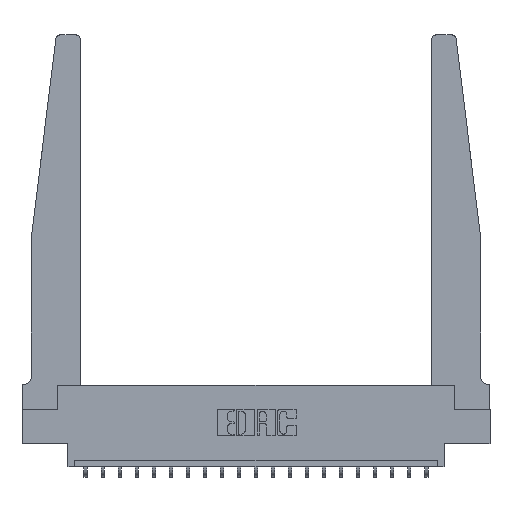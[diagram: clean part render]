
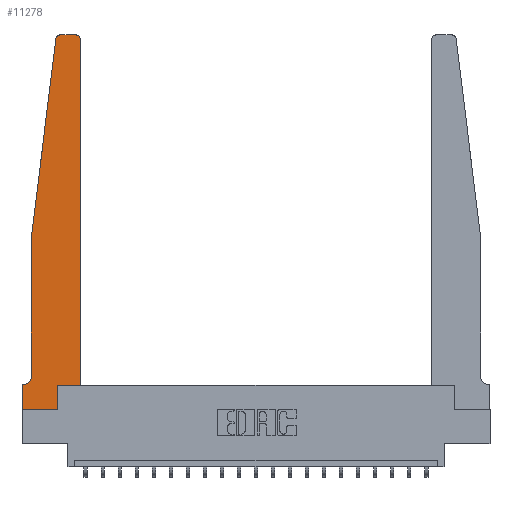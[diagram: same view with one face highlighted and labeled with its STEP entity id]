
A CAD part, top view. The second image highlights one B-rep face of the part: STEP entity #11278.
In plain terms, the highlighted planar face has unit normal (0, 0, 1).
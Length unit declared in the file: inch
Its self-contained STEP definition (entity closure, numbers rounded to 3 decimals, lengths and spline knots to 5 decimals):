
#734 = DIRECTION ( 'NONE',  ( 0., 1., 0. ) ) ;
#1067 = EDGE_CURVE ( 'NONE', #11489, #17803, #10407, .T. ) ;
#1849 = ORIENTED_EDGE ( 'NONE', *, *, #5977, .T. ) ;
#2045 = CARTESIAN_POINT ( 'NONE',  ( 0., 0., 0.37 ) ) ;
#2107 = DIRECTION ( 'NONE',  ( 0., 0., 1. ) ) ;
#2179 = ORIENTED_EDGE ( 'NONE', *, *, #11530, .T. ) ;
#2269 = AXIS2_PLACEMENT_3D ( 'NONE', #3315, #14620, #4945 ) ;
#2359 = LINE ( 'NONE', #6190, #10485 ) ;
#2527 = CARTESIAN_POINT ( 'NONE',  ( 0.2605, 0.18, 0.37 ) ) ;
#3315 = CARTESIAN_POINT ( 'NONE',  ( 0.015, 0.2375, 0.37 ) ) ;
#3487 = LINE ( 'NONE', #10428, #12092 ) ;
#3528 = CARTESIAN_POINT ( 'NONE',  ( 0.395, 2.75, 0.37 ) ) ;
#3557 = PLANE ( 'NONE',  #18861 ) ;
#3589 = VERTEX_POINT ( 'NONE', #8562 ) ;
#4024 = VERTEX_POINT ( 'NONE', #3528 ) ;
#4036 = CARTESIAN_POINT ( 'NONE',  ( 0.27653, 2.75, 0.37 ) ) ;
#4040 = ORIENTED_EDGE ( 'NONE', *, *, #19664, .T. ) ;
#4415 = CARTESIAN_POINT ( 'NONE',  ( 0., 0.1875, 0.37 ) ) ;
#4531 = DIRECTION ( 'NONE',  ( 1., 0., 0. ) ) ;
#4720 = VECTOR ( 'NONE', #15456, 39.37008 ) ;
#4945 = DIRECTION ( 'NONE',  ( -1., 0., 0. ) ) ;
#4988 = VECTOR ( 'NONE', #8500, 39.37008 ) ;
#5121 = EDGE_CURVE ( 'NONE', #16998, #19607, #2359, .T. ) ;
#5365 = DIRECTION ( 'NONE',  ( -1., 0., 0. ) ) ;
#5428 = CARTESIAN_POINT ( 'NONE',  ( 0.2605, 0., 0.37 ) ) ;
#5687 = VECTOR ( 'NONE', #20597, 39.37008 ) ;
#5770 = LINE ( 'NONE', #18410, #20823 ) ;
#5849 = ORIENTED_EDGE ( 'NONE', *, *, #1067, .T. ) ;
#5855 = ORIENTED_EDGE ( 'NONE', *, *, #16783, .T. ) ;
#5861 = EDGE_CURVE ( 'NONE', #13091, #3589, #6192, .T. ) ;
#5977 = EDGE_CURVE ( 'NONE', #15714, #17641, #16508, .T. ) ;
#5997 = LINE ( 'NONE', #6769, #14083 ) ;
#6190 = CARTESIAN_POINT ( 'NONE',  ( 0.425, 0.18, 0.37 ) ) ;
#6192 = LINE ( 'NONE', #15740, #5687 ) ;
#6405 = ORIENTED_EDGE ( 'NONE', *, *, #5861, .T. ) ;
#6511 = DIRECTION ( 'NONE',  ( -1., 0., 0. ) ) ;
#6769 = CARTESIAN_POINT ( 'NONE',  ( 0.065, 1.25, 0.37 ) ) ;
#7740 = ORIENTED_EDGE ( 'NONE', *, *, #10599, .T. ) ;
#8424 = DIRECTION ( 'NONE',  ( 1., 0., 0. ) ) ;
#8441 = VERTEX_POINT ( 'NONE', #15940 ) ;
#8500 = DIRECTION ( 'NONE',  ( 0., -1., 0. ) ) ;
#8562 = CARTESIAN_POINT ( 'NONE',  ( 0.065, 0.2375, 0.37 ) ) ;
#8772 = LINE ( 'NONE', #2045, #4988 ) ;
#9014 = AXIS2_PLACEMENT_3D ( 'NONE', #18676, #9339, #4531 ) ;
#9070 = ORIENTED_EDGE ( 'NONE', *, *, #5121, .T. ) ;
#9339 = DIRECTION ( 'NONE',  ( 0., 0., 1. ) ) ;
#9696 = CARTESIAN_POINT ( 'NONE',  ( 0.065, 0.1875, 0.37 ) ) ;
#10064 = ORIENTED_EDGE ( 'NONE', *, *, #17966, .T. ) ;
#10296 = ORIENTED_EDGE ( 'NONE', *, *, #11317, .T. ) ;
#10407 = CIRCLE ( 'NONE', #9014, 0.03 ) ;
#10428 = CARTESIAN_POINT ( 'NONE',  ( 0.425, 0.18, 0.37 ) ) ;
#10485 = VECTOR ( 'NONE', #15761, 39.37008 ) ;
#10599 = EDGE_CURVE ( 'NONE', #16716, #19806, #5770, .T. ) ;
#10815 = CARTESIAN_POINT ( 'NONE',  ( 0.2605, 0.18, 0.37 ) ) ;
#10894 = EDGE_CURVE ( 'NONE', #19607, #8441, #3487, .T. ) ;
#11007 = CIRCLE ( 'NONE', #15887, 0.03 ) ;
#11278 = ADVANCED_FACE ( 'NONE', ( #17801 ), #3557, .T. ) ;
#11317 = EDGE_CURVE ( 'NONE', #17641, #16716, #8772, .T. ) ;
#11489 = VERTEX_POINT ( 'NONE', #4036 ) ;
#11521 = ORIENTED_EDGE ( 'NONE', *, *, #19553, .T. ) ;
#11530 = EDGE_CURVE ( 'NONE', #19806, #16998, #17539, .T. ) ;
#11832 = CARTESIAN_POINT ( 'NONE',  ( 0.395, 2.72, 0.37 ) ) ;
#12092 = VECTOR ( 'NONE', #734, 39.37008 ) ;
#12973 = CARTESIAN_POINT ( 'NONE',  ( 0.065, 1.25, 0.37 ) ) ;
#13091 = VERTEX_POINT ( 'NONE', #12973 ) ;
#13451 = DIRECTION ( 'NONE',  ( 1., 0., 0. ) ) ;
#14083 = VECTOR ( 'NONE', #16408, 39.37008 ) ;
#14582 = EDGE_LOOP ( 'NONE', ( #5855, #5849, #4040, #6405, #11521, #1849, #10296, #7740, #2179, #9070, #18549, #10064 ) ) ;
#14620 = DIRECTION ( 'NONE',  ( 0., 0., -1. ) ) ;
#14892 = CARTESIAN_POINT ( 'NONE',  ( 0., 0., 0.37 ) ) ;
#15079 = CIRCLE ( 'NONE', #2269, 0.05 ) ;
#15275 = LINE ( 'NONE', #19798, #15772 ) ;
#15456 = DIRECTION ( 'NONE',  ( 0., 1., 0. ) ) ;
#15714 = VERTEX_POINT ( 'NONE', #19849 ) ;
#15740 = CARTESIAN_POINT ( 'NONE',  ( 0.065, 1.25, 0.37 ) ) ;
#15761 = DIRECTION ( 'NONE',  ( 1., 0., 0. ) ) ;
#15772 = VECTOR ( 'NONE', #5365, 39.37008 ) ;
#15887 = AXIS2_PLACEMENT_3D ( 'NONE', #11832, #2107, #13451 ) ;
#15940 = CARTESIAN_POINT ( 'NONE',  ( 0.425, 2.72, 0.37 ) ) ;
#16363 = CARTESIAN_POINT ( 'NONE',  ( 0., 0.1875, 0.37 ) ) ;
#16408 = DIRECTION ( 'NONE',  ( -0.122, -0.992, 0. ) ) ;
#16508 = LINE ( 'NONE', #9696, #20215 ) ;
#16716 = VERTEX_POINT ( 'NONE', #14892 ) ;
#16783 = EDGE_CURVE ( 'NONE', #4024, #11489, #15275, .T. ) ;
#16998 = VERTEX_POINT ( 'NONE', #10815 ) ;
#17539 = LINE ( 'NONE', #2527, #4720 ) ;
#17641 = VERTEX_POINT ( 'NONE', #4415 ) ;
#17801 = FACE_OUTER_BOUND ( 'NONE', #14582, .T. ) ;
#17803 = VERTEX_POINT ( 'NONE', #19346 ) ;
#17966 = EDGE_CURVE ( 'NONE', #8441, #4024, #11007, .T. ) ;
#18016 = DIRECTION ( 'NONE',  ( 0., 0., 1. ) ) ;
#18410 = CARTESIAN_POINT ( 'NONE',  ( 0., 0., 0.37 ) ) ;
#18549 = ORIENTED_EDGE ( 'NONE', *, *, #10894, .T. ) ;
#18676 = CARTESIAN_POINT ( 'NONE',  ( 0.27653, 2.72, 0.37 ) ) ;
#18861 = AXIS2_PLACEMENT_3D ( 'NONE', #16363, #18016, #8424 ) ;
#19346 = CARTESIAN_POINT ( 'NONE',  ( 0.24675, 2.72367, 0.37 ) ) ;
#19456 = CARTESIAN_POINT ( 'NONE',  ( 0.425, 0.18, 0.37 ) ) ;
#19553 = EDGE_CURVE ( 'NONE', #3589, #15714, #15079, .T. ) ;
#19607 = VERTEX_POINT ( 'NONE', #19456 ) ;
#19664 = EDGE_CURVE ( 'NONE', #17803, #13091, #5997, .T. ) ;
#19798 = CARTESIAN_POINT ( 'NONE',  ( 0.25, 2.75, 0.37 ) ) ;
#19806 = VERTEX_POINT ( 'NONE', #5428 ) ;
#19849 = CARTESIAN_POINT ( 'NONE',  ( 0.015, 0.1875, 0.37 ) ) ;
#20010 = DIRECTION ( 'NONE',  ( 1., 0., 0. ) ) ;
#20215 = VECTOR ( 'NONE', #6511, 39.37008 ) ;
#20597 = DIRECTION ( 'NONE',  ( 0., -1., 0. ) ) ;
#20823 = VECTOR ( 'NONE', #20010, 39.37008 ) ;
